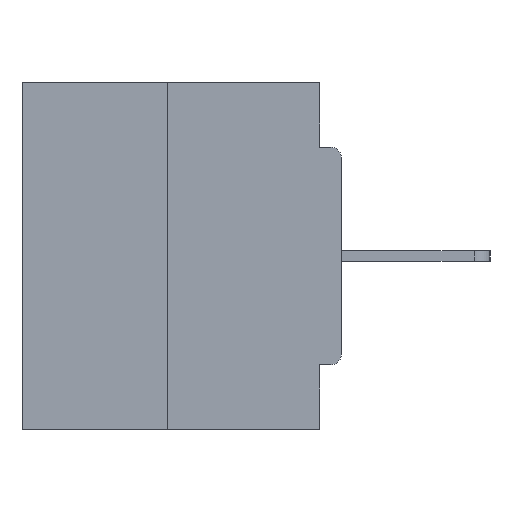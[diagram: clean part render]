
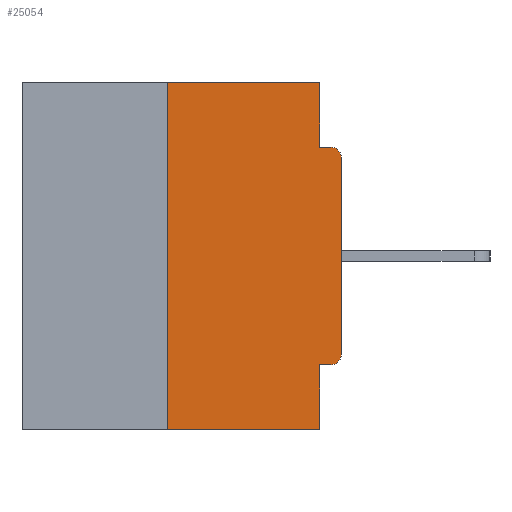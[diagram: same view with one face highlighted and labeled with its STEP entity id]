
A CAD part, left-side view. The second image highlights one B-rep face of the part: STEP entity #25054.
In plain terms, the highlighted planar face has unit normal (-1, 0, 0).
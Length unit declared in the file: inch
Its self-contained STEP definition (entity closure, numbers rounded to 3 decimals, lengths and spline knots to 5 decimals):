
#551 = AXIS2_PLACEMENT_3D ( 'NONE', #17891, #20225, #4618 ) ;
#755 = CARTESIAN_POINT ( 'NONE',  ( 0., 0.25, -0.5 ) ) ;
#1523 = ORIENTED_EDGE ( 'NONE', *, *, #27426, .T. ) ;
#1646 = ORIENTED_EDGE ( 'NONE', *, *, #2365, .F. ) ;
#1844 = DIRECTION ( 'NONE',  ( 0., 0., -1. ) ) ;
#2130 = CARTESIAN_POINT ( 'NONE',  ( 0., 0.031, -0.5 ) ) ;
#2346 = ORIENTED_EDGE ( 'NONE', *, *, #8570, .T. ) ;
#2365 = EDGE_CURVE ( 'NONE', #8626, #5653, #13581, .T. ) ;
#2399 = EDGE_CURVE ( 'NONE', #5653, #14597, #4717, .T. ) ;
#3428 = ORIENTED_EDGE ( 'NONE', *, *, #2399, .F. ) ;
#4333 = PLANE ( 'NONE',  #551 ) ;
#4618 = DIRECTION ( 'NONE',  ( 0., 0., -1. ) ) ;
#4661 = VERTEX_POINT ( 'NONE', #17194 ) ;
#4717 = LINE ( 'NONE', #13716, #4869 ) ;
#4869 = VECTOR ( 'NONE', #24440, 39.37008 ) ;
#4941 = CARTESIAN_POINT ( 'NONE',  ( 0., 0.031, 0. ) ) ;
#5653 = VERTEX_POINT ( 'NONE', #21586 ) ;
#6471 = VERTEX_POINT ( 'NONE', #21948 ) ;
#6481 = DIRECTION ( 'NONE',  ( 0., 1., 0. ) ) ;
#6909 = CARTESIAN_POINT ( 'NONE',  ( 0., 0., -0.4065 ) ) ;
#6929 = CARTESIAN_POINT ( 'NONE',  ( 0., 0.031, 0. ) ) ;
#7743 = VERTEX_POINT ( 'NONE', #17136 ) ;
#7950 = VERTEX_POINT ( 'NONE', #755 ) ;
#8076 = CARTESIAN_POINT ( 'NONE',  ( 0., 0.015, -0.1085 ) ) ;
#8296 = VECTOR ( 'NONE', #24862, 39.37008 ) ;
#8570 = EDGE_CURVE ( 'NONE', #7950, #15006, #19688, .T. ) ;
#8593 = DIRECTION ( 'NONE',  ( 0., 0., -1. ) ) ;
#8626 = VERTEX_POINT ( 'NONE', #4941 ) ;
#8828 = VECTOR ( 'NONE', #24539, 39.37008 ) ;
#9104 = ORIENTED_EDGE ( 'NONE', *, *, #23786, .T. ) ;
#9562 = CARTESIAN_POINT ( 'NONE',  ( 0., 0.25, 0. ) ) ;
#10578 = AXIS2_PLACEMENT_3D ( 'NONE', #8076, #19417, #19128 ) ;
#10846 = VECTOR ( 'NONE', #6481, 39.37008 ) ;
#11096 = DIRECTION ( 'NONE',  ( -1., 0., 0. ) ) ;
#11107 = VECTOR ( 'NONE', #14989, 39.37008 ) ;
#11370 = VECTOR ( 'NONE', #1844, 39.37008 ) ;
#13231 = CARTESIAN_POINT ( 'NONE',  ( 0., 0.46, 0. ) ) ;
#13335 = VECTOR ( 'NONE', #29039, 39.37008 ) ;
#13581 = LINE ( 'NONE', #6929, #13335 ) ;
#13716 = CARTESIAN_POINT ( 'NONE',  ( 0., 0., -0.0935 ) ) ;
#13744 = VECTOR ( 'NONE', #20989, 39.37008 ) ;
#13851 = ORIENTED_EDGE ( 'NONE', *, *, #25089, .F. ) ;
#14246 = LINE ( 'NONE', #27482, #13744 ) ;
#14417 = EDGE_CURVE ( 'NONE', #22397, #4661, #23986, .T. ) ;
#14597 = VERTEX_POINT ( 'NONE', #16978 ) ;
#14989 = DIRECTION ( 'NONE',  ( 0., -1., 0. ) ) ;
#15006 = VERTEX_POINT ( 'NONE', #18705 ) ;
#15772 = LINE ( 'NONE', #6909, #10846 ) ;
#16375 = EDGE_CURVE ( 'NONE', #7950, #24936, #27093, .T. ) ;
#16978 = CARTESIAN_POINT ( 'NONE',  ( 0., 0.015, -0.0935 ) ) ;
#17136 = CARTESIAN_POINT ( 'NONE',  ( 0., 0.031, -0.4065 ) ) ;
#17194 = CARTESIAN_POINT ( 'NONE',  ( 0., 0., -0.3915 ) ) ;
#17835 = EDGE_CURVE ( 'NONE', #24936, #8626, #24397, .T. ) ;
#17891 = CARTESIAN_POINT ( 'NONE',  ( 0., 0.46, 0. ) ) ;
#18705 = CARTESIAN_POINT ( 'NONE',  ( 0., 0.031, -0.5 ) ) ;
#19128 = DIRECTION ( 'NONE',  ( 0., 0., -1. ) ) ;
#19347 = CARTESIAN_POINT ( 'NONE',  ( 0., 0.015, -0.4065 ) ) ;
#19371 = CARTESIAN_POINT ( 'NONE',  ( 0., 0.25, 0. ) ) ;
#19417 = DIRECTION ( 'NONE',  ( -1., 0., 0. ) ) ;
#19688 = LINE ( 'NONE', #28818, #11107 ) ;
#19962 = CIRCLE ( 'NONE', #10578, 0.015 ) ;
#20188 = ORIENTED_EDGE ( 'NONE', *, *, #17835, .F. ) ;
#20225 = DIRECTION ( 'NONE',  ( 1., 0., 0. ) ) ;
#20989 = DIRECTION ( 'NONE',  ( 0., 0., 1. ) ) ;
#21441 = ORIENTED_EDGE ( 'NONE', *, *, #14417, .T. ) ;
#21544 = EDGE_LOOP ( 'NONE', ( #20188, #26827, #2346, #13851, #24220, #21441, #9104, #1523, #3428, #1646 ) ) ;
#21586 = CARTESIAN_POINT ( 'NONE',  ( 0., 0.031, -0.0935 ) ) ;
#21901 = EDGE_CURVE ( 'NONE', #22397, #7743, #15772, .T. ) ;
#21948 = CARTESIAN_POINT ( 'NONE',  ( 0., 0., -0.1085 ) ) ;
#22397 = VERTEX_POINT ( 'NONE', #19347 ) ;
#22568 = LINE ( 'NONE', #2130, #11370 ) ;
#23041 = AXIS2_PLACEMENT_3D ( 'NONE', #27143, #11096, #8593 ) ;
#23786 = EDGE_CURVE ( 'NONE', #4661, #6471, #14246, .T. ) ;
#23986 = CIRCLE ( 'NONE', #23041, 0.015 ) ;
#24220 = ORIENTED_EDGE ( 'NONE', *, *, #21901, .F. ) ;
#24341 = FACE_OUTER_BOUND ( 'NONE', #21544, .T. ) ;
#24397 = LINE ( 'NONE', #13231, #8828 ) ;
#24440 = DIRECTION ( 'NONE',  ( 0., -1., 0. ) ) ;
#24539 = DIRECTION ( 'NONE',  ( 0., -1., 0. ) ) ;
#24862 = DIRECTION ( 'NONE',  ( 0., 0., 1. ) ) ;
#24936 = VERTEX_POINT ( 'NONE', #19371 ) ;
#25054 = ADVANCED_FACE ( 'NONE', ( #24341 ), #4333, .F. ) ;
#25089 = EDGE_CURVE ( 'NONE', #7743, #15006, #22568, .T. ) ;
#26827 = ORIENTED_EDGE ( 'NONE', *, *, #16375, .F. ) ;
#27093 = LINE ( 'NONE', #9562, #8296 ) ;
#27143 = CARTESIAN_POINT ( 'NONE',  ( 0., 0.015, -0.3915 ) ) ;
#27426 = EDGE_CURVE ( 'NONE', #6471, #14597, #19962, .T. ) ;
#27482 = CARTESIAN_POINT ( 'NONE',  ( 0., 0., 0. ) ) ;
#28818 = CARTESIAN_POINT ( 'NONE',  ( 0., 0.46, -0.5 ) ) ;
#29039 = DIRECTION ( 'NONE',  ( 0., 0., -1. ) ) ;
